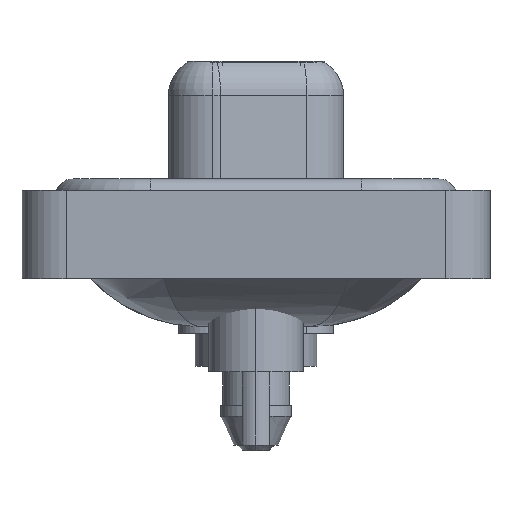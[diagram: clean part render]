
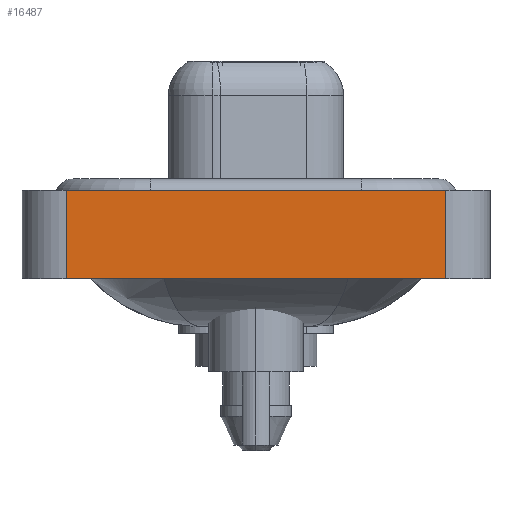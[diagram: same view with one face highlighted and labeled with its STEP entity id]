
A CAD part, left-side view. The second image highlights one B-rep face of the part: STEP entity #16487.
In plain terms, the highlighted planar face has unit normal (-1, 0, 0).
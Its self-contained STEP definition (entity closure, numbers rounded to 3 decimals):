
#667 = LINE ( 'NONE', #18245, #944 ) ;
#733 = EDGE_CURVE ( 'NONE', #8686, #17951, #6252, .T. ) ;
#944 = VECTOR ( 'NONE', #2601, 1000. ) ;
#1070 = VERTEX_POINT ( 'NONE', #6034 ) ;
#1194 = FACE_OUTER_BOUND ( 'NONE', #5061, .T. ) ;
#1568 = DIRECTION ( 'NONE',  ( 0., -1., 0. ) ) ;
#2601 = DIRECTION ( 'NONE',  ( 0., 0., 1. ) ) ;
#2647 = CARTESIAN_POINT ( 'NONE',  ( -7.3, -8.55, -3.6 ) ) ;
#2899 = VECTOR ( 'NONE', #1568, 1000. ) ;
#3435 = VERTEX_POINT ( 'NONE', #15959 ) ;
#4161 = DIRECTION ( 'NONE',  ( 0., 0., 1. ) ) ;
#4630 = CARTESIAN_POINT ( 'NONE',  ( -7.3, -8.55, 0.4 ) ) ;
#5061 = EDGE_LOOP ( 'NONE', ( #18493, #6938, #14162, #10227 ) ) ;
#6034 = CARTESIAN_POINT ( 'NONE',  ( -7.3, 8.55, -3.6 ) ) ;
#6252 = LINE ( 'NONE', #13614, #2899 ) ;
#6351 = LINE ( 'NONE', #6446, #18660 ) ;
#6446 = CARTESIAN_POINT ( 'NONE',  ( -7.3, -8.55, -3.6 ) ) ;
#6938 = ORIENTED_EDGE ( 'NONE', *, *, #733, .F. ) ;
#8686 = VERTEX_POINT ( 'NONE', #12410 ) ;
#9553 = EDGE_CURVE ( 'NONE', #1070, #8686, #667, .T. ) ;
#9617 = VECTOR ( 'NONE', #15534, 1000. ) ;
#10227 = ORIENTED_EDGE ( 'NONE', *, *, #17582, .T. ) ;
#10459 = AXIS2_PLACEMENT_3D ( 'NONE', #2647, #11522, #4161 ) ;
#11256 = CARTESIAN_POINT ( 'NONE',  ( -7.3, -8.55, -3.6 ) ) ;
#11522 = DIRECTION ( 'NONE',  ( -1., 0., 0. ) ) ;
#12410 = CARTESIAN_POINT ( 'NONE',  ( -7.3, 8.55, 0.4 ) ) ;
#12486 = LINE ( 'NONE', #11256, #9617 ) ;
#13614 = CARTESIAN_POINT ( 'NONE',  ( -7.3, -8.55, 0.4 ) ) ;
#13952 = EDGE_CURVE ( 'NONE', #3435, #17951, #6351, .T. ) ;
#14162 = ORIENTED_EDGE ( 'NONE', *, *, #9553, .F. ) ;
#14485 = PLANE ( 'NONE',  #10459 ) ;
#15534 = DIRECTION ( 'NONE',  ( 0., -1., 0. ) ) ;
#15678 = DIRECTION ( 'NONE',  ( 0., 0., 1. ) ) ;
#15959 = CARTESIAN_POINT ( 'NONE',  ( -7.3, -8.55, -3.6 ) ) ;
#16487 = ADVANCED_FACE ( 'NONE', ( #1194 ), #14485, .T. ) ;
#17582 = EDGE_CURVE ( 'NONE', #1070, #3435, #12486, .T. ) ;
#17951 = VERTEX_POINT ( 'NONE', #4630 ) ;
#18245 = CARTESIAN_POINT ( 'NONE',  ( -7.3, 8.55, -3.6 ) ) ;
#18493 = ORIENTED_EDGE ( 'NONE', *, *, #13952, .T. ) ;
#18660 = VECTOR ( 'NONE', #15678, 1000. ) ;
